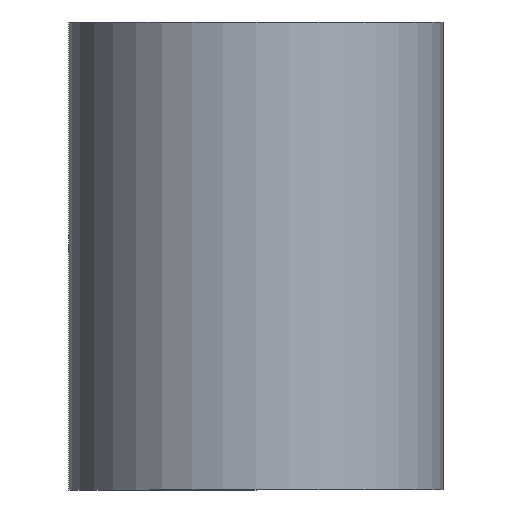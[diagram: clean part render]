
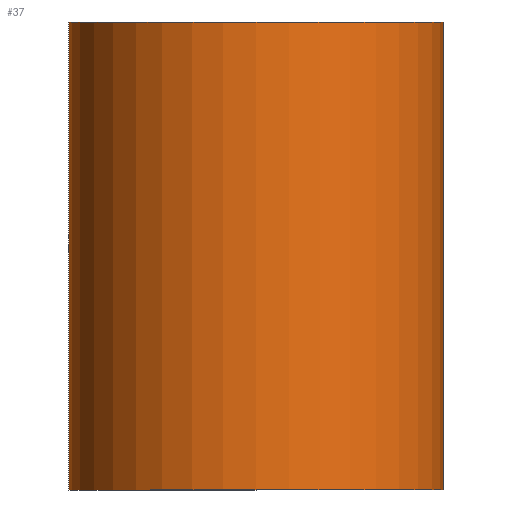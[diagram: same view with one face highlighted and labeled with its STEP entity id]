
A CAD part, left-side view. The second image highlights one B-rep face of the part: STEP entity #37.
In plain terms, the highlighted cylindrical face has radius 3 mm (diameter 6 mm), a partial arc.
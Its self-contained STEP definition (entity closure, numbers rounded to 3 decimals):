
#1 = CARTESIAN_POINT ( 'NONE',  ( 0., 0., 7.5 ) ) ;
#3 = CARTESIAN_POINT ( 'NONE',  ( 0., 3., 0. ) ) ;
#8 = AXIS2_PLACEMENT_3D ( 'NONE', #1, #12, #70 ) ;
#12 = DIRECTION ( 'NONE',  ( 0., 0., 1. ) ) ;
#17 = AXIS2_PLACEMENT_3D ( 'NONE', #96, #65, #48 ) ;
#18 = EDGE_CURVE ( 'NONE', #139, #58, #110, .T. ) ;
#20 = EDGE_CURVE ( 'NONE', #134, #58, #24, .T. ) ;
#23 = AXIS2_PLACEMENT_3D ( 'NONE', #119, #114, #28 ) ;
#24 = CIRCLE ( 'NONE', #17, 3. ) ;
#28 = DIRECTION ( 'NONE',  ( 0., 1., 0. ) ) ;
#30 = CARTESIAN_POINT ( 'NONE',  ( 0., 3., 7.5 ) ) ;
#37 = ADVANCED_FACE ( 'NONE', ( #107 ), #97, .T. ) ;
#43 = CARTESIAN_POINT ( 'NONE',  ( 0., -3., 0. ) ) ;
#47 = EDGE_CURVE ( 'NONE', #116, #134, #101, .T. ) ;
#48 = DIRECTION ( 'NONE',  ( 0., 1., 0. ) ) ;
#52 = CARTESIAN_POINT ( 'NONE',  ( 0., -3., 7.5 ) ) ;
#58 = VERTEX_POINT ( 'NONE', #3 ) ;
#61 = CARTESIAN_POINT ( 'NONE',  ( 0., 3., 7.5 ) ) ;
#65 = DIRECTION ( 'NONE',  ( 0., 0., -1. ) ) ;
#66 = ORIENTED_EDGE ( 'NONE', *, *, #86, .F. ) ;
#68 = DIRECTION ( 'NONE',  ( 0., 0., -1. ) ) ;
#70 = DIRECTION ( 'NONE',  ( 0., 1., 0. ) ) ;
#86 = EDGE_CURVE ( 'NONE', #139, #116, #87, .T. ) ;
#87 = CIRCLE ( 'NONE', #8, 3. ) ;
#90 = CARTESIAN_POINT ( 'NONE',  ( 0., -3., 7.5 ) ) ;
#93 = VECTOR ( 'NONE', #68, 1000. ) ;
#95 = ORIENTED_EDGE ( 'NONE', *, *, #47, .F. ) ;
#96 = CARTESIAN_POINT ( 'NONE',  ( 0., 0., 0. ) ) ;
#97 = CYLINDRICAL_SURFACE ( 'NONE', #23, 3. ) ;
#101 = LINE ( 'NONE', #52, #93 ) ;
#107 = FACE_OUTER_BOUND ( 'NONE', #121, .T. ) ;
#108 = VECTOR ( 'NONE', #120, 1000. ) ;
#110 = LINE ( 'NONE', #61, #108 ) ;
#112 = ORIENTED_EDGE ( 'NONE', *, *, #18, .T. ) ;
#114 = DIRECTION ( 'NONE',  ( 0., 0., -1. ) ) ;
#116 = VERTEX_POINT ( 'NONE', #90 ) ;
#119 = CARTESIAN_POINT ( 'NONE',  ( 0., 0., 7.5 ) ) ;
#120 = DIRECTION ( 'NONE',  ( 0., 0., -1. ) ) ;
#121 = EDGE_LOOP ( 'NONE', ( #95, #66, #112, #124 ) ) ;
#124 = ORIENTED_EDGE ( 'NONE', *, *, #20, .F. ) ;
#134 = VERTEX_POINT ( 'NONE', #43 ) ;
#139 = VERTEX_POINT ( 'NONE', #30 ) ;
